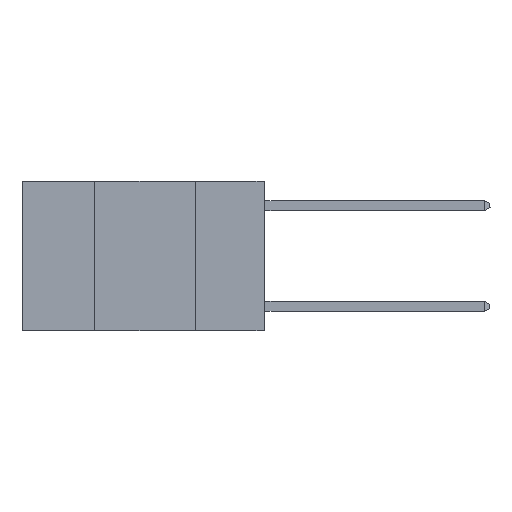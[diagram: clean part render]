
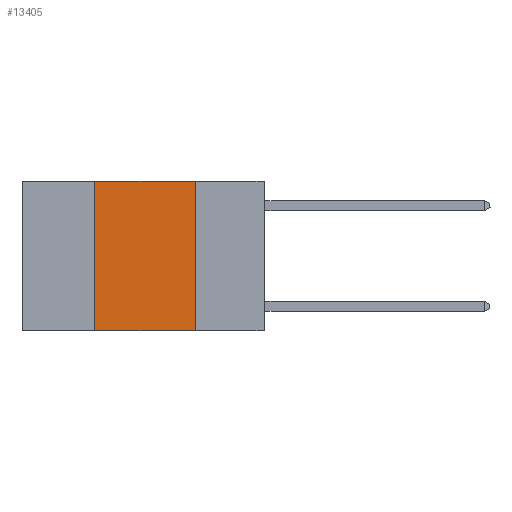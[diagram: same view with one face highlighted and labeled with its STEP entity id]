
A CAD part, left-side view. The second image highlights one B-rep face of the part: STEP entity #13405.
In plain terms, the highlighted planar face has unit normal (-1, 0, 0).
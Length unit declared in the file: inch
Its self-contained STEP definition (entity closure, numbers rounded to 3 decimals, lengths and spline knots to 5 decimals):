
#148 = PLANE ( 'NONE',  #5074 ) ;
#267 = DIRECTION ( 'NONE',  ( 0., -1., 0. ) ) ;
#1057 = VERTEX_POINT ( 'NONE', #18373 ) ;
#2384 = DIRECTION ( 'NONE',  ( 0., 0., -1. ) ) ;
#3436 = EDGE_CURVE ( 'NONE', #9998, #1057, #11045, .T. ) ;
#5074 = AXIS2_PLACEMENT_3D ( 'NONE', #8884, #15385, #2384 ) ;
#5320 = DIRECTION ( 'NONE',  ( 0., 0., -1. ) ) ;
#6440 = ORIENTED_EDGE ( 'NONE', *, *, #3436, .F. ) ;
#7811 = CARTESIAN_POINT ( 'NONE',  ( 0., 0.42, 0. ) ) ;
#8518 = ORIENTED_EDGE ( 'NONE', *, *, #15220, .T. ) ;
#8884 = CARTESIAN_POINT ( 'NONE',  ( 0., 0.6, 0. ) ) ;
#9998 = VERTEX_POINT ( 'NONE', #25592 ) ;
#10000 = DIRECTION ( 'NONE',  ( 0., 0., 1. ) ) ;
#10380 = VECTOR ( 'NONE', #19088, 39.37008 ) ;
#10889 = EDGE_CURVE ( 'NONE', #1057, #12753, #27321, .T. ) ;
#11045 = LINE ( 'NONE', #16958, #10380 ) ;
#11978 = VECTOR ( 'NONE', #267, 39.37008 ) ;
#12753 = VERTEX_POINT ( 'NONE', #13444 ) ;
#13405 = ADVANCED_FACE ( 'NONE', ( #23947 ), #148, .F. ) ;
#13444 = CARTESIAN_POINT ( 'NONE',  ( 0., 0.17, -0.37 ) ) ;
#13778 = EDGE_CURVE ( 'NONE', #20376, #9998, #15419, .T. ) ;
#15220 = EDGE_CURVE ( 'NONE', #20376, #12753, #23211, .T. ) ;
#15385 = DIRECTION ( 'NONE',  ( 1., 0., 0. ) ) ;
#15419 = LINE ( 'NONE', #7811, #24563 ) ;
#16958 = CARTESIAN_POINT ( 'NONE',  ( 0., 0.6, 0. ) ) ;
#17959 = ORIENTED_EDGE ( 'NONE', *, *, #13778, .F. ) ;
#18373 = CARTESIAN_POINT ( 'NONE',  ( 0., 0.17, 0. ) ) ;
#19088 = DIRECTION ( 'NONE',  ( 0., -1., 0. ) ) ;
#20272 = CARTESIAN_POINT ( 'NONE',  ( 0., 0.17, 0. ) ) ;
#20376 = VERTEX_POINT ( 'NONE', #20526 ) ;
#20526 = CARTESIAN_POINT ( 'NONE',  ( 0., 0.42, -0.37 ) ) ;
#21838 = CARTESIAN_POINT ( 'NONE',  ( 0., 0.6, -0.37 ) ) ;
#23211 = LINE ( 'NONE', #21838, #11978 ) ;
#23786 = ORIENTED_EDGE ( 'NONE', *, *, #10889, .F. ) ;
#23947 = FACE_OUTER_BOUND ( 'NONE', #24532, .T. ) ;
#24532 = EDGE_LOOP ( 'NONE', ( #23786, #6440, #17959, #8518 ) ) ;
#24563 = VECTOR ( 'NONE', #10000, 39.37008 ) ;
#25592 = CARTESIAN_POINT ( 'NONE',  ( 0., 0.42, 0. ) ) ;
#26660 = VECTOR ( 'NONE', #5320, 39.37008 ) ;
#27321 = LINE ( 'NONE', #20272, #26660 ) ;
